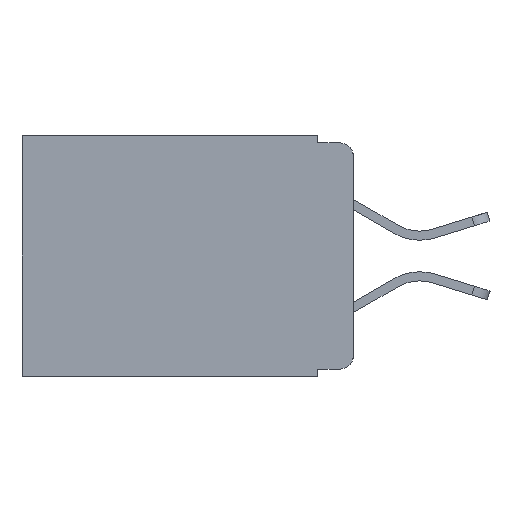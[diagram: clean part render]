
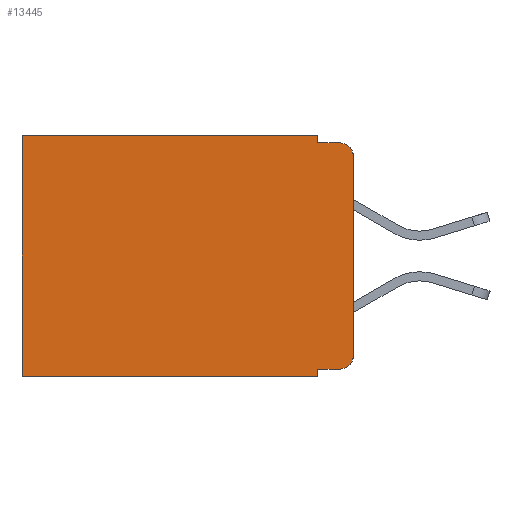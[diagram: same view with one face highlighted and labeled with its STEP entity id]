
A CAD part, left-side view. The second image highlights one B-rep face of the part: STEP entity #13445.
In plain terms, the highlighted planar face has unit normal (-1, 0, 0).
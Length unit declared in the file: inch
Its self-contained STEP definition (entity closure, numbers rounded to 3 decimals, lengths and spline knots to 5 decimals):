
#103 = VECTOR ( 'NONE', #608, 39.37008 ) ;
#391 = CARTESIAN_POINT ( 'NONE',  ( 0.298, 0.051, -0.333 ) ) ;
#565 = LINE ( 'NONE', #12811, #865 ) ;
#608 = DIRECTION ( 'NONE',  ( 0., 0., -1. ) ) ;
#639 = EDGE_CURVE ( 'NONE', #9013, #24622, #3519, .T. ) ;
#865 = VECTOR ( 'NONE', #20683, 39.37008 ) ;
#984 = LINE ( 'NONE', #14790, #8494 ) ;
#1010 = ORIENTED_EDGE ( 'NONE', *, *, #3674, .F. ) ;
#1217 = ORIENTED_EDGE ( 'NONE', *, *, #9410, .T. ) ;
#1469 = VERTEX_POINT ( 'NONE', #10530 ) ;
#1485 = ORIENTED_EDGE ( 'NONE', *, *, #7406, .F. ) ;
#1773 = ORIENTED_EDGE ( 'NONE', *, *, #8551, .F. ) ;
#1857 = CARTESIAN_POINT ( 'NONE',  ( 0.298, 0.051, -0.01 ) ) ;
#2222 = CARTESIAN_POINT ( 'NONE',  ( 0.298, 0., 0. ) ) ;
#2312 = AXIS2_PLACEMENT_3D ( 'NONE', #12435, #4591, #10477 ) ;
#2522 = CARTESIAN_POINT ( 'NONE',  ( 0.298, 0.473, 0. ) ) ;
#3490 = ORIENTED_EDGE ( 'NONE', *, *, #18545, .F. ) ;
#3519 = LINE ( 'NONE', #19246, #10940 ) ;
#3674 = EDGE_CURVE ( 'NONE', #18704, #1469, #4153, .T. ) ;
#3684 = VERTEX_POINT ( 'NONE', #8050 ) ;
#4113 = EDGE_CURVE ( 'NONE', #16641, #3684, #9825, .T. ) ;
#4153 = LINE ( 'NONE', #12505, #20584 ) ;
#4178 = LINE ( 'NONE', #2222, #24027 ) ;
#4400 = CIRCLE ( 'NONE', #2312, 0.02 ) ;
#4412 = DIRECTION ( 'NONE',  ( 0., 0., -1. ) ) ;
#4591 = DIRECTION ( 'NONE',  ( -1., 0., 0. ) ) ;
#5077 = AXIS2_PLACEMENT_3D ( 'NONE', #13997, #5646, #21755 ) ;
#5376 = VERTEX_POINT ( 'NONE', #18354 ) ;
#5634 = CARTESIAN_POINT ( 'NONE',  ( 0.298, 0.051, -0.01 ) ) ;
#5646 = DIRECTION ( 'NONE',  ( 1., 0., 0. ) ) ;
#5795 = CARTESIAN_POINT ( 'NONE',  ( 0.298, 0.473, -0.343 ) ) ;
#6495 = ORIENTED_EDGE ( 'NONE', *, *, #18449, .F. ) ;
#7284 = VERTEX_POINT ( 'NONE', #13737 ) ;
#7406 = EDGE_CURVE ( 'NONE', #5376, #22109, #565, .T. ) ;
#7852 = CARTESIAN_POINT ( 'NONE',  ( 0.298, 0.051, -0.333 ) ) ;
#8050 = CARTESIAN_POINT ( 'NONE',  ( 0.298, 0., -0.313 ) ) ;
#8494 = VECTOR ( 'NONE', #22836, 39.37008 ) ;
#8551 = EDGE_CURVE ( 'NONE', #9650, #3684, #14149, .T. ) ;
#8809 = LINE ( 'NONE', #391, #23441 ) ;
#9013 = VERTEX_POINT ( 'NONE', #2522 ) ;
#9410 = EDGE_CURVE ( 'NONE', #5376, #9013, #4178, .T. ) ;
#9650 = VERTEX_POINT ( 'NONE', #13163 ) ;
#9684 = ORIENTED_EDGE ( 'NONE', *, *, #4113, .T. ) ;
#9825 = CIRCLE ( 'NONE', #24335, 0.02 ) ;
#10176 = DIRECTION ( 'NONE',  ( 0., 1., 0. ) ) ;
#10477 = DIRECTION ( 'NONE',  ( 0., 0., -1. ) ) ;
#10530 = CARTESIAN_POINT ( 'NONE',  ( 0.298, 0.051, -0.343 ) ) ;
#10940 = VECTOR ( 'NONE', #21570, 39.37008 ) ;
#11404 = FACE_OUTER_BOUND ( 'NONE', #12462, .T. ) ;
#12225 = DIRECTION ( 'NONE',  ( 0., 0., -1. ) ) ;
#12435 = CARTESIAN_POINT ( 'NONE',  ( 0.298, 0.02, -0.03 ) ) ;
#12462 = EDGE_LOOP ( 'NONE', ( #1773, #18975, #3490, #1485, #1217, #24896, #6495, #1010, #20735, #9684 ) ) ;
#12505 = CARTESIAN_POINT ( 'NONE',  ( 0.298, 0.051, 0. ) ) ;
#12811 = CARTESIAN_POINT ( 'NONE',  ( 0.298, 0.051, 0. ) ) ;
#13163 = CARTESIAN_POINT ( 'NONE',  ( 0.298, 0., -0.03 ) ) ;
#13445 = ADVANCED_FACE ( 'NONE', ( #11404 ), #19816, .F. ) ;
#13737 = CARTESIAN_POINT ( 'NONE',  ( 0.298, 0.02, -0.01 ) ) ;
#13997 = CARTESIAN_POINT ( 'NONE',  ( 0.298, 0., 0. ) ) ;
#14149 = LINE ( 'NONE', #24153, #103 ) ;
#14790 = CARTESIAN_POINT ( 'NONE',  ( 0.298, 0., -0.343 ) ) ;
#16641 = VERTEX_POINT ( 'NONE', #17064 ) ;
#16816 = EDGE_CURVE ( 'NONE', #18704, #16641, #8809, .T. ) ;
#17064 = CARTESIAN_POINT ( 'NONE',  ( 0.298, 0.02, -0.333 ) ) ;
#18354 = CARTESIAN_POINT ( 'NONE',  ( 0.298, 0.051, 0. ) ) ;
#18449 = EDGE_CURVE ( 'NONE', #1469, #24622, #984, .T. ) ;
#18545 = EDGE_CURVE ( 'NONE', #22109, #7284, #23095, .T. ) ;
#18704 = VERTEX_POINT ( 'NONE', #7852 ) ;
#18975 = ORIENTED_EDGE ( 'NONE', *, *, #25545, .T. ) ;
#19246 = CARTESIAN_POINT ( 'NONE',  ( 0.298, 0.473, 0. ) ) ;
#19734 = VECTOR ( 'NONE', #21495, 39.37008 ) ;
#19816 = PLANE ( 'NONE',  #5077 ) ;
#20584 = VECTOR ( 'NONE', #4412, 39.37008 ) ;
#20683 = DIRECTION ( 'NONE',  ( 0., 0., -1. ) ) ;
#20735 = ORIENTED_EDGE ( 'NONE', *, *, #16816, .T. ) ;
#21495 = DIRECTION ( 'NONE',  ( 0., -1., 0. ) ) ;
#21570 = DIRECTION ( 'NONE',  ( 0., 0., -1. ) ) ;
#21755 = DIRECTION ( 'NONE',  ( 0., 0., -1. ) ) ;
#22069 = CARTESIAN_POINT ( 'NONE',  ( 0.298, 0.02, -0.313 ) ) ;
#22109 = VERTEX_POINT ( 'NONE', #1857 ) ;
#22195 = DIRECTION ( 'NONE',  ( -1., 0., 0. ) ) ;
#22466 = DIRECTION ( 'NONE',  ( 0., -1., 0. ) ) ;
#22836 = DIRECTION ( 'NONE',  ( 0., 1., 0. ) ) ;
#23095 = LINE ( 'NONE', #5634, #19734 ) ;
#23441 = VECTOR ( 'NONE', #22466, 39.37008 ) ;
#24027 = VECTOR ( 'NONE', #10176, 39.37008 ) ;
#24153 = CARTESIAN_POINT ( 'NONE',  ( 0.298, 0., 0. ) ) ;
#24335 = AXIS2_PLACEMENT_3D ( 'NONE', #22069, #22195, #12225 ) ;
#24622 = VERTEX_POINT ( 'NONE', #5795 ) ;
#24896 = ORIENTED_EDGE ( 'NONE', *, *, #639, .T. ) ;
#25545 = EDGE_CURVE ( 'NONE', #9650, #7284, #4400, .T. ) ;
